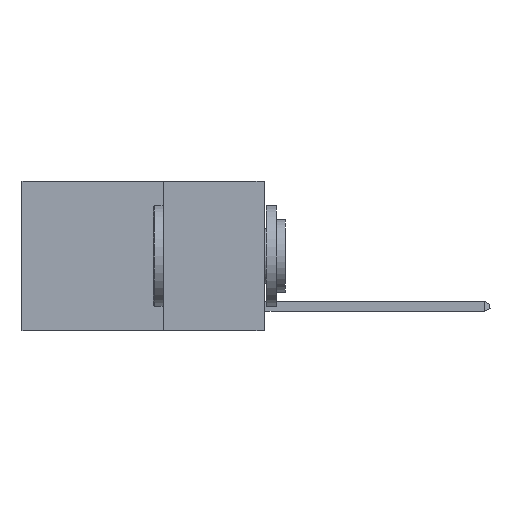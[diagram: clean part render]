
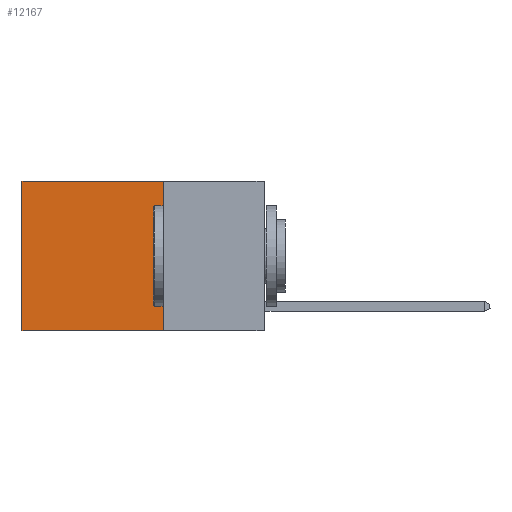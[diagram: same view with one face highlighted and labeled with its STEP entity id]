
A CAD part, left-side view. The second image highlights one B-rep face of the part: STEP entity #12167.
In plain terms, the highlighted planar face has unit normal (-1, 0, 0).
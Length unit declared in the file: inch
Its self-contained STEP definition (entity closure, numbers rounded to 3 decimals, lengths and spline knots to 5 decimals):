
#1653 = DIRECTION ( 'NONE',  ( 1., 0., 0. ) ) ;
#2429 = EDGE_CURVE ( 'NONE', #14244, #11938, #17087, .T. ) ;
#2697 = EDGE_CURVE ( 'NONE', #4335, #25889, #10584, .T. ) ;
#2776 = ORIENTED_EDGE ( 'NONE', *, *, #2429, .F. ) ;
#4335 = VERTEX_POINT ( 'NONE', #5675 ) ;
#5675 = CARTESIAN_POINT ( 'NONE',  ( 0.2625, 0.6, 0. ) ) ;
#5964 = DIRECTION ( 'NONE',  ( 0., 1., 0. ) ) ;
#7977 = FACE_OUTER_BOUND ( 'NONE', #21256, .T. ) ;
#10584 = LINE ( 'NONE', #12618, #18070 ) ;
#11284 = DIRECTION ( 'NONE',  ( 0., 0., -1. ) ) ;
#11938 = VERTEX_POINT ( 'NONE', #12631 ) ;
#12167 = ADVANCED_FACE ( 'NONE', ( #7977 ), #14206, .F. ) ;
#12488 = VECTOR ( 'NONE', #13168, 39.37008 ) ;
#12618 = CARTESIAN_POINT ( 'NONE',  ( 0.2625, 0.6, 0. ) ) ;
#12631 = CARTESIAN_POINT ( 'NONE',  ( 0.2625, 0.25, -0.37 ) ) ;
#13065 = ORIENTED_EDGE ( 'NONE', *, *, #15450, .F. ) ;
#13168 = DIRECTION ( 'NONE',  ( 0., 1., 0. ) ) ;
#13395 = EDGE_CURVE ( 'NONE', #14244, #4335, #22714, .T. ) ;
#14206 = PLANE ( 'NONE',  #17154 ) ;
#14244 = VERTEX_POINT ( 'NONE', #20355 ) ;
#15450 = EDGE_CURVE ( 'NONE', #11938, #25889, #19227, .T. ) ;
#17087 = LINE ( 'NONE', #21655, #23294 ) ;
#17154 = AXIS2_PLACEMENT_3D ( 'NONE', #24608, #1653, #18661 ) ;
#18070 = VECTOR ( 'NONE', #20832, 39.37008 ) ;
#18661 = DIRECTION ( 'NONE',  ( 0., 0., -1. ) ) ;
#19227 = LINE ( 'NONE', #21121, #12488 ) ;
#20355 = CARTESIAN_POINT ( 'NONE',  ( 0.2625, 0.25, 0. ) ) ;
#20683 = ORIENTED_EDGE ( 'NONE', *, *, #13395, .T. ) ;
#20832 = DIRECTION ( 'NONE',  ( 0., 0., -1. ) ) ;
#21121 = CARTESIAN_POINT ( 'NONE',  ( 0.2625, 0.25, -0.37 ) ) ;
#21256 = EDGE_LOOP ( 'NONE', ( #24284, #13065, #2776, #20683 ) ) ;
#21655 = CARTESIAN_POINT ( 'NONE',  ( 0.2625, 0.25, 0. ) ) ;
#22714 = LINE ( 'NONE', #24483, #23181 ) ;
#22834 = CARTESIAN_POINT ( 'NONE',  ( 0.2625, 0.6, -0.37 ) ) ;
#23181 = VECTOR ( 'NONE', #5964, 39.37008 ) ;
#23294 = VECTOR ( 'NONE', #11284, 39.37008 ) ;
#24284 = ORIENTED_EDGE ( 'NONE', *, *, #2697, .T. ) ;
#24483 = CARTESIAN_POINT ( 'NONE',  ( 0.2625, 0.25, 0. ) ) ;
#24608 = CARTESIAN_POINT ( 'NONE',  ( 0.2625, 0.25, 0. ) ) ;
#25889 = VERTEX_POINT ( 'NONE', #22834 ) ;
